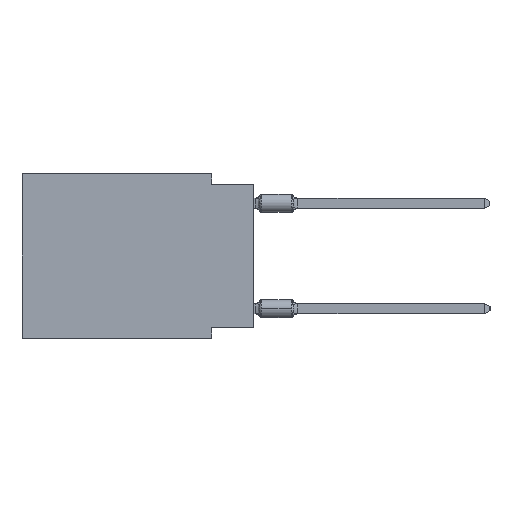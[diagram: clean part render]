
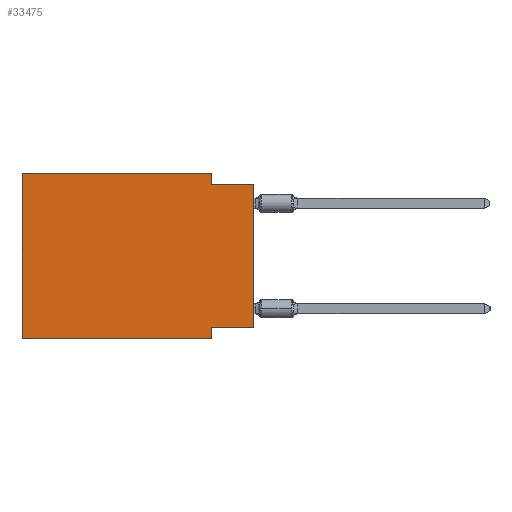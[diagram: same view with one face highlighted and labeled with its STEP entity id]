
A CAD part, left-side view. The second image highlights one B-rep face of the part: STEP entity #33475.
In plain terms, the highlighted planar face has unit normal (-1, 0, 0).
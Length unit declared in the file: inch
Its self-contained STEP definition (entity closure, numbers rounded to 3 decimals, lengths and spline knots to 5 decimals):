
#1234 = LINE ( 'NONE', #22226, #7260 ) ;
#1354 = DIRECTION ( 'NONE',  ( 0., -1., 0. ) ) ;
#1612 = VERTEX_POINT ( 'NONE', #14191 ) ;
#2199 = DIRECTION ( 'NONE',  ( 0., 0., 1. ) ) ;
#2750 = LINE ( 'NONE', #31042, #21532 ) ;
#3001 = VECTOR ( 'NONE', #2199, 39.37008 ) ;
#3472 = CARTESIAN_POINT ( 'NONE',  ( 0., 0.55, 0. ) ) ;
#4986 = DIRECTION ( 'NONE',  ( 0., -1., 0. ) ) ;
#5610 = CARTESIAN_POINT ( 'NONE',  ( 0., 0., -0.365 ) ) ;
#7260 = VECTOR ( 'NONE', #4986, 39.37008 ) ;
#7733 = CARTESIAN_POINT ( 'NONE',  ( 0., 0.55, 0. ) ) ;
#7904 = EDGE_CURVE ( 'NONE', #19074, #11180, #24002, .T. ) ;
#8812 = LINE ( 'NONE', #34724, #3001 ) ;
#9390 = VERTEX_POINT ( 'NONE', #3472 ) ;
#9592 = DIRECTION ( 'NONE',  ( 0., 0., 1. ) ) ;
#10267 = ORIENTED_EDGE ( 'NONE', *, *, #39313, .F. ) ;
#10305 = EDGE_CURVE ( 'NONE', #16726, #42125, #1234, .T. ) ;
#10406 = VECTOR ( 'NONE', #30507, 39.37008 ) ;
#10784 = ORIENTED_EDGE ( 'NONE', *, *, #10305, .T. ) ;
#11180 = VERTEX_POINT ( 'NONE', #19667 ) ;
#14191 = CARTESIAN_POINT ( 'NONE',  ( 0., 0., -0.025 ) ) ;
#14590 = ORIENTED_EDGE ( 'NONE', *, *, #16980, .F. ) ;
#15164 = VERTEX_POINT ( 'NONE', #34049 ) ;
#16363 = LINE ( 'NONE', #45383, #10406 ) ;
#16726 = VERTEX_POINT ( 'NONE', #43948 ) ;
#16980 = EDGE_CURVE ( 'NONE', #15164, #1612, #24550, .T. ) ;
#19074 = VERTEX_POINT ( 'NONE', #30114 ) ;
#19370 = ORIENTED_EDGE ( 'NONE', *, *, #28659, .F. ) ;
#19667 = CARTESIAN_POINT ( 'NONE',  ( 0., 0.1, -0.365 ) ) ;
#20381 = AXIS2_PLACEMENT_3D ( 'NONE', #46382, #38629, #35785 ) ;
#20980 = ORIENTED_EDGE ( 'NONE', *, *, #7904, .F. ) ;
#21532 = VECTOR ( 'NONE', #9592, 39.37008 ) ;
#21884 = LINE ( 'NONE', #7733, #44433 ) ;
#21912 = LINE ( 'NONE', #43135, #31458 ) ;
#22226 = CARTESIAN_POINT ( 'NONE',  ( 0., 0.55, -0.39 ) ) ;
#24002 = LINE ( 'NONE', #5610, #41166 ) ;
#24550 = LINE ( 'NONE', #35640, #43828 ) ;
#24767 = EDGE_LOOP ( 'NONE', ( #27914, #14590, #19370, #31898, #10267, #10784, #43741, #20980 ) ) ;
#24828 = CARTESIAN_POINT ( 'NONE',  ( 0., 0.1, -0.39 ) ) ;
#25682 = DIRECTION ( 'NONE',  ( 0., 0., -1. ) ) ;
#27914 = ORIENTED_EDGE ( 'NONE', *, *, #46048, .T. ) ;
#28005 = FACE_OUTER_BOUND ( 'NONE', #24767, .T. ) ;
#28659 = EDGE_CURVE ( 'NONE', #43904, #15164, #16363, .T. ) ;
#28769 = CARTESIAN_POINT ( 'NONE',  ( 0., 0.1, 0. ) ) ;
#30114 = CARTESIAN_POINT ( 'NONE',  ( 0., 0., -0.365 ) ) ;
#30507 = DIRECTION ( 'NONE',  ( 0., 0., -1. ) ) ;
#31042 = CARTESIAN_POINT ( 'NONE',  ( 0., 0.55, 0. ) ) ;
#31458 = VECTOR ( 'NONE', #25682, 39.37008 ) ;
#31898 = ORIENTED_EDGE ( 'NONE', *, *, #45729, .F. ) ;
#33475 = ADVANCED_FACE ( 'NONE', ( #28005 ), #42394, .F. ) ;
#34049 = CARTESIAN_POINT ( 'NONE',  ( 0., 0.1, -0.025 ) ) ;
#34724 = CARTESIAN_POINT ( 'NONE',  ( 0., 0., 0. ) ) ;
#34932 = DIRECTION ( 'NONE',  ( 0., -1., 0. ) ) ;
#35640 = CARTESIAN_POINT ( 'NONE',  ( 0., 0., -0.025 ) ) ;
#35785 = DIRECTION ( 'NONE',  ( 0., 0., -1. ) ) ;
#38629 = DIRECTION ( 'NONE',  ( 1., 0., 0. ) ) ;
#39313 = EDGE_CURVE ( 'NONE', #16726, #9390, #2750, .T. ) ;
#41166 = VECTOR ( 'NONE', #46150, 39.37008 ) ;
#41507 = EDGE_CURVE ( 'NONE', #11180, #42125, #21912, .T. ) ;
#42125 = VERTEX_POINT ( 'NONE', #24828 ) ;
#42394 = PLANE ( 'NONE',  #20381 ) ;
#43135 = CARTESIAN_POINT ( 'NONE',  ( 0., 0.1, -0.39 ) ) ;
#43741 = ORIENTED_EDGE ( 'NONE', *, *, #41507, .F. ) ;
#43828 = VECTOR ( 'NONE', #34932, 39.37008 ) ;
#43904 = VERTEX_POINT ( 'NONE', #28769 ) ;
#43948 = CARTESIAN_POINT ( 'NONE',  ( 0., 0.55, -0.39 ) ) ;
#44433 = VECTOR ( 'NONE', #1354, 39.37008 ) ;
#45383 = CARTESIAN_POINT ( 'NONE',  ( 0., 0.1, 0. ) ) ;
#45729 = EDGE_CURVE ( 'NONE', #9390, #43904, #21884, .T. ) ;
#46048 = EDGE_CURVE ( 'NONE', #19074, #1612, #8812, .T. ) ;
#46150 = DIRECTION ( 'NONE',  ( 0., 1., 0. ) ) ;
#46382 = CARTESIAN_POINT ( 'NONE',  ( 0., 0.55, 0. ) ) ;
